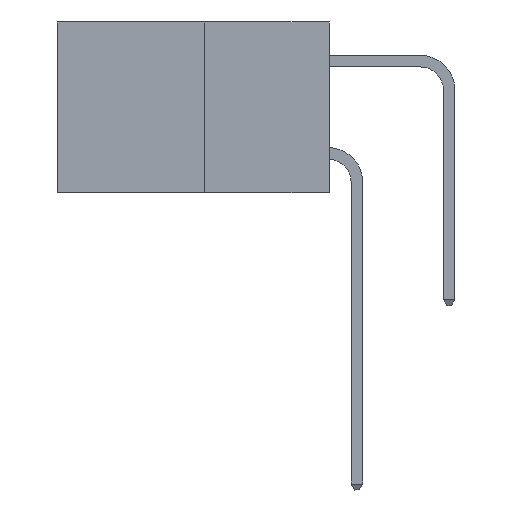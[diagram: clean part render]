
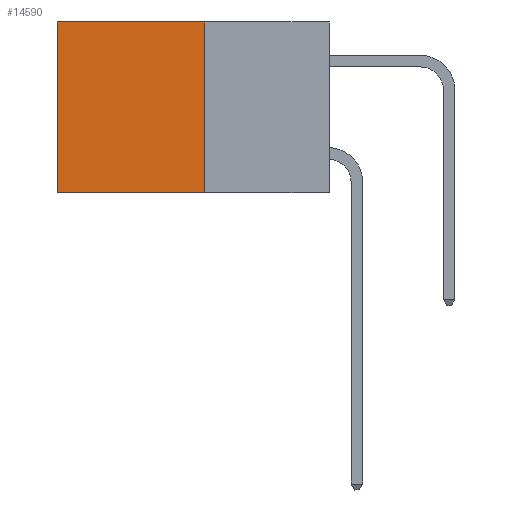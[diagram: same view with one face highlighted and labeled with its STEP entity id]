
A CAD part, left-side view. The second image highlights one B-rep face of the part: STEP entity #14590.
In plain terms, the highlighted planar face has unit normal (-1, 0, 0).
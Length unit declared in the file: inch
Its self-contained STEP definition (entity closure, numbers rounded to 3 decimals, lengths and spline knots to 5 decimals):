
#69 = LINE ( 'NONE', #7391, #25000 ) ;
#1535 = VECTOR ( 'NONE', #5412, 39.37008 ) ;
#1655 = ORIENTED_EDGE ( 'NONE', *, *, #3487, .F. ) ;
#1859 = EDGE_CURVE ( 'NONE', #29614, #28540, #16136, .T. ) ;
#2081 = AXIS2_PLACEMENT_3D ( 'NONE', #9041, #4204, #13698 ) ;
#2412 = VECTOR ( 'NONE', #26549, 39.37008 ) ;
#3027 = CARTESIAN_POINT ( 'NONE',  ( 0.277, 0.27, 0. ) ) ;
#3487 = EDGE_CURVE ( 'NONE', #17686, #22674, #26576, .T. ) ;
#4204 = DIRECTION ( 'NONE',  ( 1., 0., 0. ) ) ;
#5412 = DIRECTION ( 'NONE',  ( 0., 1., 0. ) ) ;
#7112 = CARTESIAN_POINT ( 'NONE',  ( 0.277, 0.59, -0.37 ) ) ;
#7391 = CARTESIAN_POINT ( 'NONE',  ( 0.277, 0.27, -0.37 ) ) ;
#7726 = EDGE_LOOP ( 'NONE', ( #25211, #10524, #1655, #12678 ) ) ;
#7867 = LINE ( 'NONE', #3027, #1535 ) ;
#9041 = CARTESIAN_POINT ( 'NONE',  ( 0.277, 0.27, -0.37 ) ) ;
#10524 = ORIENTED_EDGE ( 'NONE', *, *, #17485, .F. ) ;
#11369 = PLANE ( 'NONE',  #2081 ) ;
#11880 = CARTESIAN_POINT ( 'NONE',  ( 0.277, 0.27, -0.37 ) ) ;
#12678 = ORIENTED_EDGE ( 'NONE', *, *, #19582, .T. ) ;
#12751 = CARTESIAN_POINT ( 'NONE',  ( 0.277, 0.27, 0. ) ) ;
#13698 = DIRECTION ( 'NONE',  ( 0., 0., -1. ) ) ;
#14590 = ADVANCED_FACE ( 'NONE', ( #23683 ), #11369, .F. ) ;
#16136 = LINE ( 'NONE', #17219, #29192 ) ;
#17219 = CARTESIAN_POINT ( 'NONE',  ( 0.277, 0.59, -0.37 ) ) ;
#17485 = EDGE_CURVE ( 'NONE', #22674, #28540, #69, .T. ) ;
#17686 = VERTEX_POINT ( 'NONE', #12751 ) ;
#19582 = EDGE_CURVE ( 'NONE', #17686, #29614, #7867, .T. ) ;
#22674 = VERTEX_POINT ( 'NONE', #11880 ) ;
#23592 = DIRECTION ( 'NONE',  ( 0., 1., 0. ) ) ;
#23683 = FACE_OUTER_BOUND ( 'NONE', #7726, .T. ) ;
#24757 = CARTESIAN_POINT ( 'NONE',  ( 0.277, 0.59, 0. ) ) ;
#25000 = VECTOR ( 'NONE', #23592, 39.37008 ) ;
#25041 = CARTESIAN_POINT ( 'NONE',  ( 0.277, 0.27, -0.37 ) ) ;
#25211 = ORIENTED_EDGE ( 'NONE', *, *, #1859, .T. ) ;
#26549 = DIRECTION ( 'NONE',  ( 0., 0., -1. ) ) ;
#26576 = LINE ( 'NONE', #25041, #2412 ) ;
#28540 = VERTEX_POINT ( 'NONE', #7112 ) ;
#29192 = VECTOR ( 'NONE', #30009, 39.37008 ) ;
#29614 = VERTEX_POINT ( 'NONE', #24757 ) ;
#30009 = DIRECTION ( 'NONE',  ( 0., 0., -1. ) ) ;
